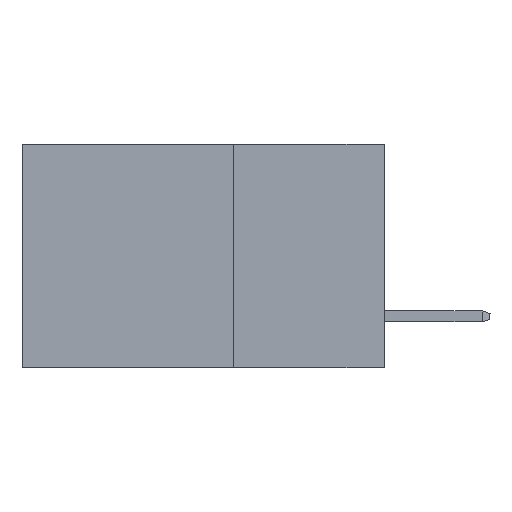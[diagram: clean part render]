
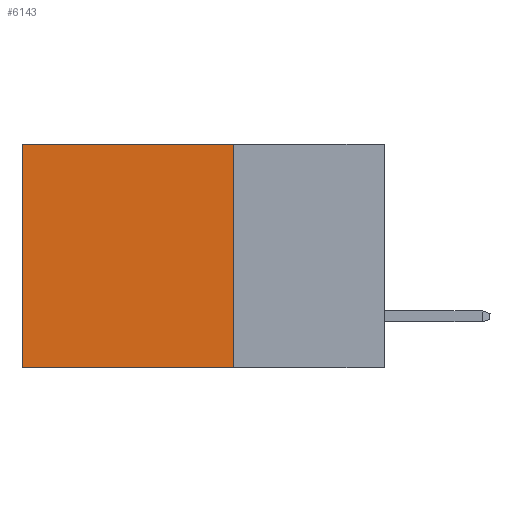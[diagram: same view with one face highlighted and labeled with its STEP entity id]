
A CAD part, left-side view. The second image highlights one B-rep face of the part: STEP entity #6143.
In plain terms, the highlighted planar face has unit normal (-1, 0, 0).
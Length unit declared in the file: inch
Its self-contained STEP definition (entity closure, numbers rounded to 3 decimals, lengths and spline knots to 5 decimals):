
#77 = ORIENTED_EDGE ( 'NONE', *, *, #4524, .T. ) ;
#84 = CARTESIAN_POINT ( 'NONE',  ( 0.2615, 0.25, -0.37 ) ) ;
#118 = CARTESIAN_POINT ( 'NONE',  ( 0.2615, 0.6, -0.37 ) ) ;
#497 = VERTEX_POINT ( 'NONE', #84 ) ;
#523 = CARTESIAN_POINT ( 'NONE',  ( 0.2615, 0.25, -0.37 ) ) ;
#823 = VECTOR ( 'NONE', #3545, 39.37008 ) ;
#1259 = CARTESIAN_POINT ( 'NONE',  ( 0.2615, 0.25, -0.37 ) ) ;
#1411 = VERTEX_POINT ( 'NONE', #6152 ) ;
#1985 = CARTESIAN_POINT ( 'NONE',  ( 0.2615, 0.25, 0. ) ) ;
#2105 = DIRECTION ( 'NONE',  ( 1., 0., 0. ) ) ;
#2318 = LINE ( 'NONE', #523, #7475 ) ;
#2434 = VECTOR ( 'NONE', #4066, 39.37008 ) ;
#2664 = EDGE_CURVE ( 'NONE', #4020, #497, #7551, .T. ) ;
#2939 = EDGE_CURVE ( 'NONE', #4020, #7285, #6470, .T. ) ;
#3545 = DIRECTION ( 'NONE',  ( 0., 0., -1. ) ) ;
#3841 = EDGE_LOOP ( 'NONE', ( #77, #9244, #9098, #6681 ) ) ;
#4020 = VERTEX_POINT ( 'NONE', #5006 ) ;
#4066 = DIRECTION ( 'NONE',  ( 0., 0., -1. ) ) ;
#4229 = CARTESIAN_POINT ( 'NONE',  ( 0.2615, 0.6, 0. ) ) ;
#4328 = LINE ( 'NONE', #118, #823 ) ;
#4524 = EDGE_CURVE ( 'NONE', #7285, #1411, #4328, .T. ) ;
#4985 = DIRECTION ( 'NONE',  ( 0., 1., 0. ) ) ;
#5006 = CARTESIAN_POINT ( 'NONE',  ( 0.2615, 0.25, 0. ) ) ;
#5522 = DIRECTION ( 'NONE',  ( 0., 0., -1. ) ) ;
#5771 = FACE_OUTER_BOUND ( 'NONE', #3841, .T. ) ;
#6143 = ADVANCED_FACE ( 'NONE', ( #5771 ), #6364, .F. ) ;
#6152 = CARTESIAN_POINT ( 'NONE',  ( 0.2615, 0.6, -0.37 ) ) ;
#6364 = PLANE ( 'NONE',  #10096 ) ;
#6470 = LINE ( 'NONE', #1985, #9943 ) ;
#6681 = ORIENTED_EDGE ( 'NONE', *, *, #2939, .T. ) ;
#7285 = VERTEX_POINT ( 'NONE', #4229 ) ;
#7475 = VECTOR ( 'NONE', #4985, 39.37008 ) ;
#7551 = LINE ( 'NONE', #9141, #2434 ) ;
#7564 = EDGE_CURVE ( 'NONE', #497, #1411, #2318, .T. ) ;
#8920 = DIRECTION ( 'NONE',  ( 0., 1., 0. ) ) ;
#9098 = ORIENTED_EDGE ( 'NONE', *, *, #2664, .F. ) ;
#9141 = CARTESIAN_POINT ( 'NONE',  ( 0.2615, 0.25, -0.37 ) ) ;
#9244 = ORIENTED_EDGE ( 'NONE', *, *, #7564, .F. ) ;
#9943 = VECTOR ( 'NONE', #8920, 39.37008 ) ;
#10096 = AXIS2_PLACEMENT_3D ( 'NONE', #1259, #2105, #5522 ) ;
